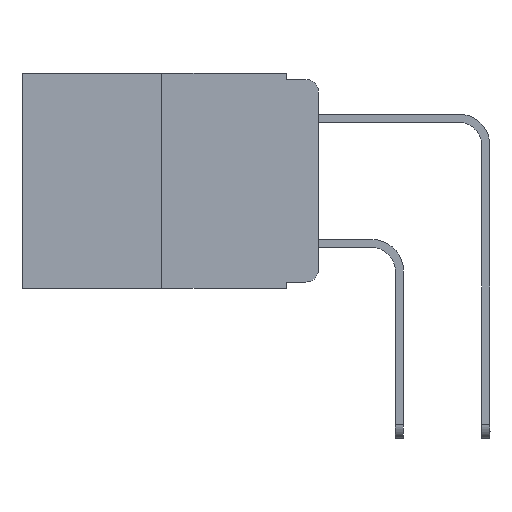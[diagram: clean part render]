
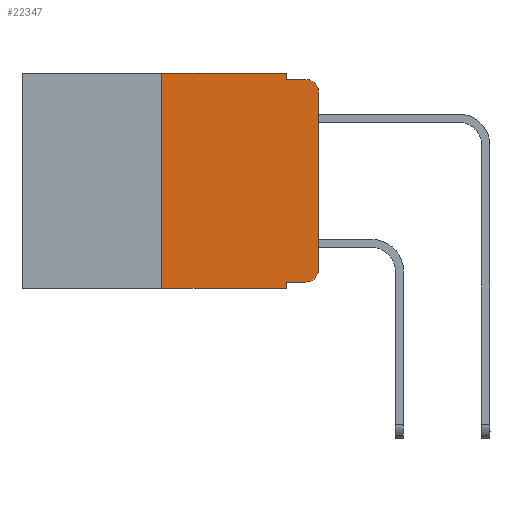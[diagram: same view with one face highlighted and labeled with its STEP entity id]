
A CAD part, left-side view. The second image highlights one B-rep face of the part: STEP entity #22347.
In plain terms, the highlighted planar face has unit normal (-1, 0, 0).
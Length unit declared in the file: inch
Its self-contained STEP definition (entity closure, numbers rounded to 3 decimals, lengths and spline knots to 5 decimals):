
#456 = ORIENTED_EDGE ( 'NONE', *, *, #20808, .F. ) ;
#592 = CARTESIAN_POINT ( 'NONE',  ( 0., 0.051, -0.333 ) ) ;
#1189 = CIRCLE ( 'NONE', #20636, 0.02 ) ;
#1224 = EDGE_CURVE ( 'NONE', #11130, #10407, #17574, .T. ) ;
#2589 = VERTEX_POINT ( 'NONE', #6735 ) ;
#2664 = CARTESIAN_POINT ( 'NONE',  ( 0., 0.25, 0. ) ) ;
#2754 = LINE ( 'NONE', #11183, #23673 ) ;
#2807 = CARTESIAN_POINT ( 'NONE',  ( 0., 0.02, -0.03 ) ) ;
#3246 = CARTESIAN_POINT ( 'NONE',  ( 0., 0.25, -0.343 ) ) ;
#3532 = EDGE_LOOP ( 'NONE', ( #9206, #15040, #3739, #16770, #456, #11427, #24382, #6902, #5484, #16702 ) ) ;
#3739 = ORIENTED_EDGE ( 'NONE', *, *, #21897, .F. ) ;
#4148 = EDGE_CURVE ( 'NONE', #11506, #6198, #5271, .T. ) ;
#4259 = EDGE_CURVE ( 'NONE', #5654, #2589, #1189, .T. ) ;
#4578 = VECTOR ( 'NONE', #10882, 39.37008 ) ;
#4657 = EDGE_CURVE ( 'NONE', #18633, #19449, #11451, .T. ) ;
#4895 = PLANE ( 'NONE',  #23574 ) ;
#4901 = LINE ( 'NONE', #23849, #14831 ) ;
#5024 = DIRECTION ( 'NONE',  ( 0., 0., -1. ) ) ;
#5085 = CARTESIAN_POINT ( 'NONE',  ( 0., 0.051, -0.01 ) ) ;
#5271 = LINE ( 'NONE', #20442, #25067 ) ;
#5424 = FACE_OUTER_BOUND ( 'NONE', #3532, .T. ) ;
#5484 = ORIENTED_EDGE ( 'NONE', *, *, #12795, .T. ) ;
#5536 = DIRECTION ( 'NONE',  ( 0., 0., -1. ) ) ;
#5654 = VERTEX_POINT ( 'NONE', #22949 ) ;
#6198 = VERTEX_POINT ( 'NONE', #10866 ) ;
#6261 = VECTOR ( 'NONE', #13171, 39.37008 ) ;
#6735 = CARTESIAN_POINT ( 'NONE',  ( 0., 0., -0.313 ) ) ;
#6902 = ORIENTED_EDGE ( 'NONE', *, *, #4148, .F. ) ;
#7314 = DIRECTION ( 'NONE',  ( 0., 0., -1. ) ) ;
#7343 = CARTESIAN_POINT ( 'NONE',  ( 0., 0.473, 0. ) ) ;
#8246 = VERTEX_POINT ( 'NONE', #11689 ) ;
#8838 = CARTESIAN_POINT ( 'NONE',  ( 0., 0.25, 0. ) ) ;
#9101 = EDGE_CURVE ( 'NONE', #11130, #6198, #2754, .T. ) ;
#9206 = ORIENTED_EDGE ( 'NONE', *, *, #21923, .T. ) ;
#9326 = LINE ( 'NONE', #17788, #4578 ) ;
#10407 = VERTEX_POINT ( 'NONE', #2664 ) ;
#10866 = CARTESIAN_POINT ( 'NONE',  ( 0., 0.051, -0.343 ) ) ;
#10882 = DIRECTION ( 'NONE',  ( 0., 0., 1. ) ) ;
#10919 = VECTOR ( 'NONE', #20519, 39.37008 ) ;
#10947 = CIRCLE ( 'NONE', #26413, 0.02 ) ;
#10960 = LINE ( 'NONE', #25628, #6261 ) ;
#11029 = DIRECTION ( 'NONE',  ( 0., -1., 0. ) ) ;
#11130 = VERTEX_POINT ( 'NONE', #3246 ) ;
#11183 = CARTESIAN_POINT ( 'NONE',  ( 0., 0.473, -0.343 ) ) ;
#11427 = ORIENTED_EDGE ( 'NONE', *, *, #1224, .F. ) ;
#11451 = LINE ( 'NONE', #14025, #10919 ) ;
#11506 = VERTEX_POINT ( 'NONE', #592 ) ;
#11689 = CARTESIAN_POINT ( 'NONE',  ( 0., 0., -0.03 ) ) ;
#12295 = VERTEX_POINT ( 'NONE', #14466 ) ;
#12514 = VECTOR ( 'NONE', #11029, 39.37008 ) ;
#12795 = EDGE_CURVE ( 'NONE', #11506, #5654, #4901, .T. ) ;
#13171 = DIRECTION ( 'NONE',  ( 0., -1., 0. ) ) ;
#14025 = CARTESIAN_POINT ( 'NONE',  ( 0., 0.051, 0. ) ) ;
#14466 = CARTESIAN_POINT ( 'NONE',  ( 0., 0.02, -0.01 ) ) ;
#14831 = VECTOR ( 'NONE', #21199, 39.37008 ) ;
#15040 = ORIENTED_EDGE ( 'NONE', *, *, #15399, .T. ) ;
#15399 = EDGE_CURVE ( 'NONE', #8246, #12295, #10947, .T. ) ;
#16702 = ORIENTED_EDGE ( 'NONE', *, *, #4259, .T. ) ;
#16770 = ORIENTED_EDGE ( 'NONE', *, *, #4657, .F. ) ;
#17550 = DIRECTION ( 'NONE',  ( 0., -1., 0. ) ) ;
#17574 = LINE ( 'NONE', #8838, #25292 ) ;
#17668 = LINE ( 'NONE', #5085, #12514 ) ;
#17788 = CARTESIAN_POINT ( 'NONE',  ( 0., 0., 0. ) ) ;
#18633 = VERTEX_POINT ( 'NONE', #20451 ) ;
#19449 = VERTEX_POINT ( 'NONE', #20242 ) ;
#20242 = CARTESIAN_POINT ( 'NONE',  ( 0., 0.051, -0.01 ) ) ;
#20316 = DIRECTION ( 'NONE',  ( -1., 0., 0. ) ) ;
#20442 = CARTESIAN_POINT ( 'NONE',  ( 0., 0.051, 0. ) ) ;
#20451 = CARTESIAN_POINT ( 'NONE',  ( 0., 0.051, 0. ) ) ;
#20519 = DIRECTION ( 'NONE',  ( 0., 0., -1. ) ) ;
#20636 = AXIS2_PLACEMENT_3D ( 'NONE', #24473, #20316, #5536 ) ;
#20808 = EDGE_CURVE ( 'NONE', #10407, #18633, #10960, .T. ) ;
#21199 = DIRECTION ( 'NONE',  ( 0., -1., 0. ) ) ;
#21740 = DIRECTION ( 'NONE',  ( 0., 0., -1. ) ) ;
#21748 = DIRECTION ( 'NONE',  ( -1., 0., 0. ) ) ;
#21897 = EDGE_CURVE ( 'NONE', #19449, #12295, #17668, .T. ) ;
#21923 = EDGE_CURVE ( 'NONE', #2589, #8246, #9326, .T. ) ;
#22018 = DIRECTION ( 'NONE',  ( 1., 0., 0. ) ) ;
#22347 = ADVANCED_FACE ( 'NONE', ( #5424 ), #4895, .F. ) ;
#22949 = CARTESIAN_POINT ( 'NONE',  ( 0., 0.02, -0.333 ) ) ;
#23574 = AXIS2_PLACEMENT_3D ( 'NONE', #7343, #22018, #21740 ) ;
#23673 = VECTOR ( 'NONE', #17550, 39.37008 ) ;
#23849 = CARTESIAN_POINT ( 'NONE',  ( 0., 0.051, -0.333 ) ) ;
#24382 = ORIENTED_EDGE ( 'NONE', *, *, #9101, .T. ) ;
#24473 = CARTESIAN_POINT ( 'NONE',  ( 0., 0.02, -0.313 ) ) ;
#25067 = VECTOR ( 'NONE', #7314, 39.37008 ) ;
#25292 = VECTOR ( 'NONE', #26016, 39.37008 ) ;
#25628 = CARTESIAN_POINT ( 'NONE',  ( 0., 0.473, 0. ) ) ;
#26016 = DIRECTION ( 'NONE',  ( 0., 0., 1. ) ) ;
#26413 = AXIS2_PLACEMENT_3D ( 'NONE', #2807, #21748, #5024 ) ;
